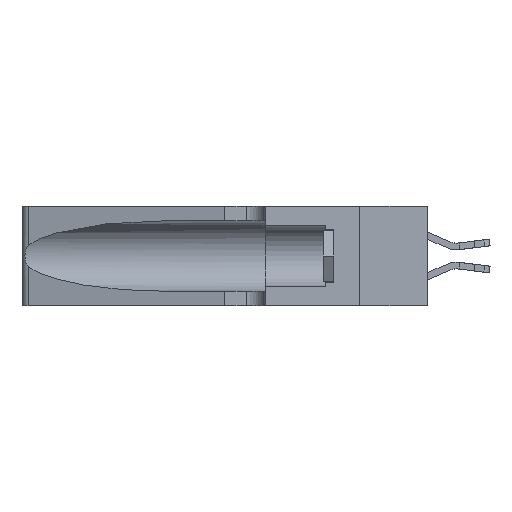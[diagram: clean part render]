
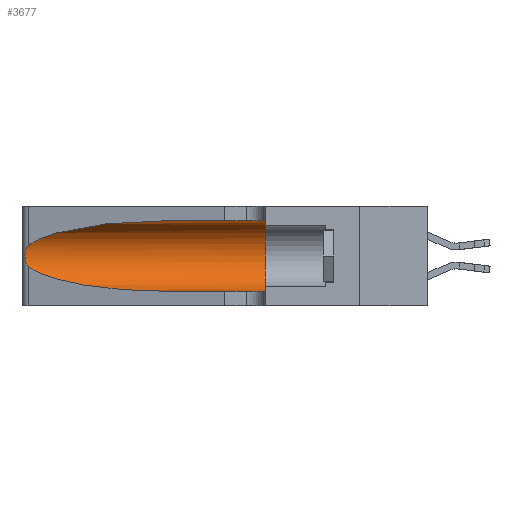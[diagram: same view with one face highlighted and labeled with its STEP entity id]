
A CAD part, left-side view. The second image highlights one B-rep face of the part: STEP entity #3677.
In plain terms, the highlighted cylindrical face has radius 3.308 mm (diameter 6.617 mm), a partial arc.
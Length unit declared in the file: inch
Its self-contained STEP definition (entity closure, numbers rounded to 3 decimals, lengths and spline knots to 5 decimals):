
#363 = ORIENTED_EDGE ( 'NONE', *, *, #19309, .F. ) ;
#846 = CARTESIAN_POINT ( 'NONE',  ( 0.1305, 0.35, 0.31525 ) ) ;
#1495 = CARTESIAN_POINT ( 'NONE',  ( 0.25639, 1.23186, 0.15144 ) ) ;
#2085 = CARTESIAN_POINT ( 'NONE',  ( 0.25487, 1.22718, 0.22369 ) ) ;
#2190 = VERTEX_POINT ( 'NONE', #27411 ) ;
#2430 = CARTESIAN_POINT ( 'NONE',  ( 0.18966, 0.96281, 0.05475 ) ) ;
#3228 = CARTESIAN_POINT ( 'NONE',  ( 0.1305, 1.61858, 0.05475 ) ) ;
#3300 = DIRECTION ( 'NONE',  ( 0., 0., 1. ) ) ;
#3677 = ADVANCED_FACE ( 'NONE', ( #6545 ), #29393, .F. ) ;
#3837 = ORIENTED_EDGE ( 'NONE', *, *, #13939, .T. ) ;
#4654 = AXIS2_PLACEMENT_3D ( 'NONE', #16240, #18516, #15842 ) ;
#4660 = CARTESIAN_POINT ( 'NONE',  ( 0.2373, 1.15595, 0.08982 ) ) ;
#5509 = CARTESIAN_POINT ( 'NONE',  ( 0.1305, 0.72297, 0.05475 ) ) ;
#6435 = VECTOR ( 'NONE', #27838, 39.37008 ) ;
#6545 = FACE_OUTER_BOUND ( 'NONE', #9179, .T. ) ;
#6685 = CARTESIAN_POINT ( 'NONE',  ( 0.25487, 1.22718, 0.14631 ) ) ;
#6849 = CARTESIAN_POINT ( 'NONE',  ( 0.25487, 1.22718, 0.14631 ) ) ;
#7033 = CIRCLE ( 'NONE', #23747, 0.13025 ) ;
#7129 = CARTESIAN_POINT ( 'NONE',  ( 0.1305, 1.61858, 0.31525 ) ) ;
#7285 = VERTEX_POINT ( 'NONE', #846 ) ;
#8104 = CARTESIAN_POINT ( 'NONE',  ( 0.25555, 1.22993, 0.14849 ) ) ;
#8196 = CARTESIAN_POINT ( 'NONE',  ( 0.1305, 0.72297, 0.31525 ) ) ;
#8197 = CARTESIAN_POINT ( 'NONE',  ( 0.26075, 1.23896, 0.178 ) ) ;
#8301 = CARTESIAN_POINT ( 'NONE',  ( 0.25487, 1.22718, 0.14631 ) ) ;
#8924 = CARTESIAN_POINT ( 'NONE',  ( 0.1305, 0.72297, 0.05475 ) ) ;
#9179 = EDGE_LOOP ( 'NONE', ( #14638, #14175, #14916, #3837, #12154, #363 ) ) ;
#9889 = DIRECTION ( 'NONE',  ( 0., -1., 0. ) ) ;
#10374 = CARTESIAN_POINT ( 'NONE',  ( 0.25854, 1.2359, 0.20912 ) ) ;
#11198 = CARTESIAN_POINT ( 'NONE',  ( 0.1305, 0.35, 0.05475 ) ) ;
#11985 = CARTESIAN_POINT ( 'NONE',  ( 0.1305, 0.72297, 0.31525 ) ) ;
#12154 = ORIENTED_EDGE ( 'NONE', *, *, #27854, .F. ) ;
#12431 = DIRECTION ( 'NONE',  ( 0., 1., 0. ) ) ;
#12675 = CARTESIAN_POINT ( 'NONE',  ( 0.25856, 1.23593, 0.16098 ) ) ;
#13939 = EDGE_CURVE ( 'NONE', #17056, #18471, #21015, .T. ) ;
#14175 = ORIENTED_EDGE ( 'NONE', *, *, #23729, .T. ) ;
#14638 = ORIENTED_EDGE ( 'NONE', *, *, #17682, .T. ) ;
#14916 = ORIENTED_EDGE ( 'NONE', *, *, #15151, .T. ) ;
#15151 = EDGE_CURVE ( 'NONE', #26526, #17056, #21774, .T. ) ;
#15222 = CARTESIAN_POINT ( 'NONE',  ( 0.25639, 1.23184, 0.21858 ) ) ;
#15842 = DIRECTION ( 'NONE',  ( 0., 0., -1. ) ) ;
#16240 = CARTESIAN_POINT ( 'NONE',  ( 0.1305, 1.61858, 0.185 ) ) ;
#17056 = VERTEX_POINT ( 'NONE', #5509 ) ;
#17189 = CARTESIAN_POINT ( 'NONE',  ( 0.25787, 1.23484, 0.2124 ) ) ;
#17487 = CARTESIAN_POINT ( 'NONE',  ( 0.26017, 1.23833, 0.17102 ) ) ;
#17682 = EDGE_CURVE ( 'NONE', #20687, #2190, #18659, .T. ) ;
#17738 = B_SPLINE_CURVE_WITH_KNOTS ( 'NONE', 3,
 ( #21897, #26317, #15222, #17189, #10374, #24131, #28546, #8197, #17487, #12675, #26421, #1495, #8104, #8301 ),
 .UNSPECIFIED., .F., .F.,
 ( 4, 2, 2, 2, 2, 2, 4 ),
 ( 0., 0.00027, 0.00053, 0.00107, 0.0016, 0.00187, 0.00214 ),
 .UNSPECIFIED. ) ;
#18471 = VERTEX_POINT ( 'NONE', #11198 ) ;
#18516 = DIRECTION ( 'NONE',  ( 0., -1., 0. ) ) ;
#18659 =( BOUNDED_CURVE ( )  B_SPLINE_CURVE ( 3, ( #8196, #28836, #26821, #2085 ),
 .UNSPECIFIED., .F., .F. ) 
 B_SPLINE_CURVE_WITH_KNOTS ( ( 4, 4 ),
 ( 1.5708, 2.84003 ),
 .UNSPECIFIED. ) 
 CURVE ( )  GEOMETRIC_REPRESENTATION_ITEM ( )  RATIONAL_B_SPLINE_CURVE ( ( 1., 0.87, 0.87, 1. ) ) 
 REPRESENTATION_ITEM ( '' )  );
#19309 = EDGE_CURVE ( 'NONE', #20687, #7285, #21683, .T. ) ;
#20687 = VERTEX_POINT ( 'NONE', #11985 ) ;
#21015 = LINE ( 'NONE', #3228, #26780 ) ;
#21683 = LINE ( 'NONE', #7129, #6435 ) ;
#21774 =( BOUNDED_CURVE ( )  B_SPLINE_CURVE ( 3, ( #6849, #4660, #2430, #8924 ),
 .UNSPECIFIED., .F., .F. ) 
 B_SPLINE_CURVE_WITH_KNOTS ( ( 4, 4 ),
 ( 3.44316, 4.71239 ),
 .UNSPECIFIED. ) 
 CURVE ( )  GEOMETRIC_REPRESENTATION_ITEM ( )  RATIONAL_B_SPLINE_CURVE ( ( 1., 0.87, 0.87, 1. ) ) 
 REPRESENTATION_ITEM ( '' )  );
#21897 = CARTESIAN_POINT ( 'NONE',  ( 0.25487, 1.22718, 0.22369 ) ) ;
#23729 = EDGE_CURVE ( 'NONE', #2190, #26526, #17738, .T. ) ;
#23747 = AXIS2_PLACEMENT_3D ( 'NONE', #28418, #12431, #3300 ) ;
#24131 = CARTESIAN_POINT ( 'NONE',  ( 0.26018, 1.23835, 0.19895 ) ) ;
#26317 = CARTESIAN_POINT ( 'NONE',  ( 0.25555, 1.22994, 0.2215 ) ) ;
#26421 = CARTESIAN_POINT ( 'NONE',  ( 0.25789, 1.23486, 0.15765 ) ) ;
#26526 = VERTEX_POINT ( 'NONE', #6685 ) ;
#26780 = VECTOR ( 'NONE', #9889, 39.37008 ) ;
#26821 = CARTESIAN_POINT ( 'NONE',  ( 0.2373, 1.15595, 0.28018 ) ) ;
#27411 = CARTESIAN_POINT ( 'NONE',  ( 0.25487, 1.22718, 0.22369 ) ) ;
#27838 = DIRECTION ( 'NONE',  ( 0., -1., 0. ) ) ;
#27854 = EDGE_CURVE ( 'NONE', #7285, #18471, #7033, .T. ) ;
#28418 = CARTESIAN_POINT ( 'NONE',  ( 0.1305, 0.35, 0.185 ) ) ;
#28546 = CARTESIAN_POINT ( 'NONE',  ( 0.26075, 1.23896, 0.19203 ) ) ;
#28836 = CARTESIAN_POINT ( 'NONE',  ( 0.18966, 0.96281, 0.31525 ) ) ;
#29393 = CYLINDRICAL_SURFACE ( 'NONE', #4654, 0.13025 ) ;
